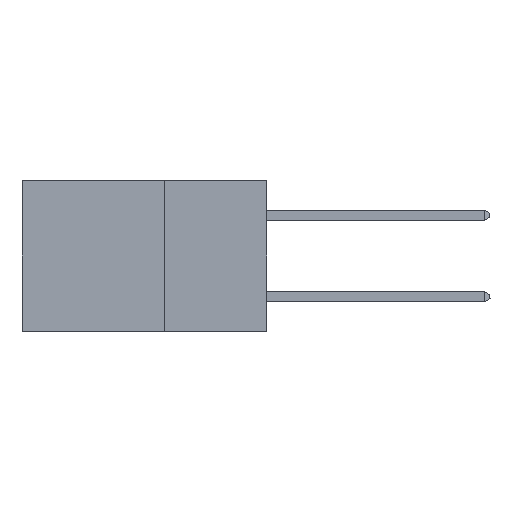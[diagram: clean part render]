
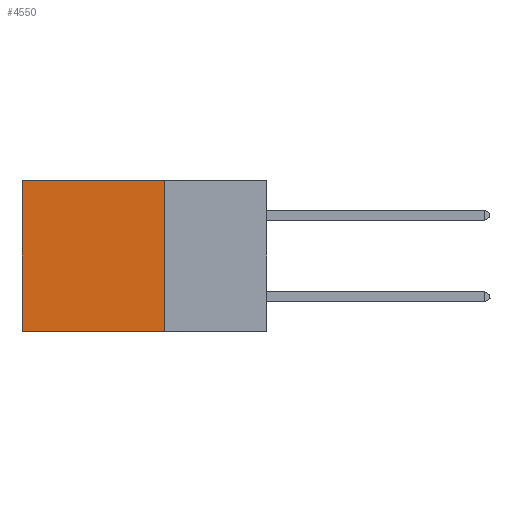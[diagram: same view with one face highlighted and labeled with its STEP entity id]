
A CAD part, left-side view. The second image highlights one B-rep face of the part: STEP entity #4550.
In plain terms, the highlighted planar face has unit normal (-1, 0, 0).
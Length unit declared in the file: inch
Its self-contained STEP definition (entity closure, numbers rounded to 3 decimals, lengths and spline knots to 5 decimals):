
#757 = VECTOR ( 'NONE', #8112, 39.37008 ) ;
#826 = EDGE_CURVE ( 'NONE', #22302, #12949, #10453, .T. ) ;
#1858 = CARTESIAN_POINT ( 'NONE',  ( 0.2875, 0.25, 0. ) ) ;
#2275 = CARTESIAN_POINT ( 'NONE',  ( 0.2875, 0.25, -0.37 ) ) ;
#2413 = LINE ( 'NONE', #3475, #757 ) ;
#3475 = CARTESIAN_POINT ( 'NONE',  ( 0.2875, 0.6, 0. ) ) ;
#3522 = CARTESIAN_POINT ( 'NONE',  ( 0.2875, 0.25, 0. ) ) ;
#4550 = ADVANCED_FACE ( 'NONE', ( #22406 ), #16764, .F. ) ;
#5985 = DIRECTION ( 'NONE',  ( 0., 0., -1. ) ) ;
#6307 = ORIENTED_EDGE ( 'NONE', *, *, #826, .F. ) ;
#6525 = EDGE_CURVE ( 'NONE', #27764, #22302, #20312, .T. ) ;
#7563 = CARTESIAN_POINT ( 'NONE',  ( 0.2875, 0.25, -0.37 ) ) ;
#8112 = DIRECTION ( 'NONE',  ( 0., 0., -1. ) ) ;
#8561 = ORIENTED_EDGE ( 'NONE', *, *, #18376, .T. ) ;
#10453 = LINE ( 'NONE', #7563, #27686 ) ;
#10663 = CARTESIAN_POINT ( 'NONE',  ( 0.2875, 0.25, 0. ) ) ;
#11989 = VECTOR ( 'NONE', #18785, 39.37008 ) ;
#11991 = DIRECTION ( 'NONE',  ( 0., 1., 0. ) ) ;
#12949 = VERTEX_POINT ( 'NONE', #21087 ) ;
#13257 = CARTESIAN_POINT ( 'NONE',  ( 0.2875, 0.6, 0. ) ) ;
#13335 = ORIENTED_EDGE ( 'NONE', *, *, #6525, .F. ) ;
#13339 = EDGE_CURVE ( 'NONE', #22373, #12949, #2413, .T. ) ;
#13633 = AXIS2_PLACEMENT_3D ( 'NONE', #3522, #18922, #5985 ) ;
#14354 = CARTESIAN_POINT ( 'NONE',  ( 0.2875, 0.25, 0. ) ) ;
#16764 = PLANE ( 'NONE',  #13633 ) ;
#18376 = EDGE_CURVE ( 'NONE', #27764, #22373, #25137, .T. ) ;
#18785 = DIRECTION ( 'NONE',  ( 0., 1., 0. ) ) ;
#18922 = DIRECTION ( 'NONE',  ( 1., 0., 0. ) ) ;
#19251 = DIRECTION ( 'NONE',  ( 0., 0., -1. ) ) ;
#19642 = VECTOR ( 'NONE', #19251, 39.37008 ) ;
#19979 = ORIENTED_EDGE ( 'NONE', *, *, #13339, .T. ) ;
#20201 = EDGE_LOOP ( 'NONE', ( #19979, #6307, #13335, #8561 ) ) ;
#20312 = LINE ( 'NONE', #1858, #19642 ) ;
#21087 = CARTESIAN_POINT ( 'NONE',  ( 0.2875, 0.6, -0.37 ) ) ;
#22302 = VERTEX_POINT ( 'NONE', #2275 ) ;
#22373 = VERTEX_POINT ( 'NONE', #13257 ) ;
#22406 = FACE_OUTER_BOUND ( 'NONE', #20201, .T. ) ;
#25137 = LINE ( 'NONE', #14354, #11989 ) ;
#27686 = VECTOR ( 'NONE', #11991, 39.37008 ) ;
#27764 = VERTEX_POINT ( 'NONE', #10663 ) ;
